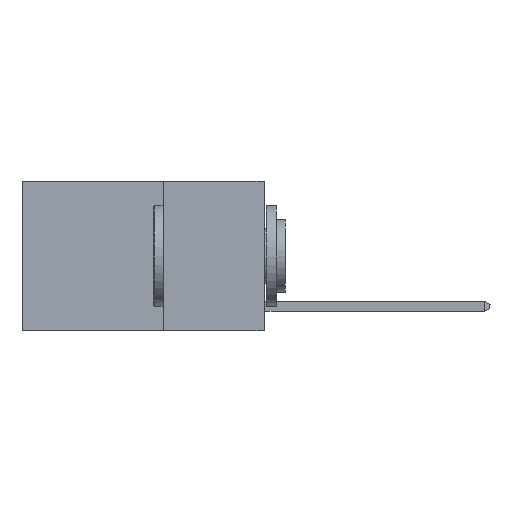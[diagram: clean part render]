
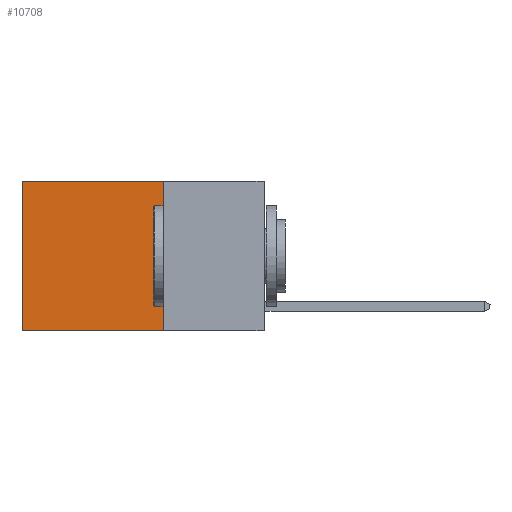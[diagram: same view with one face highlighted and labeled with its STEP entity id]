
A CAD part, left-side view. The second image highlights one B-rep face of the part: STEP entity #10708.
In plain terms, the highlighted planar face has unit normal (-1, 0, 0).
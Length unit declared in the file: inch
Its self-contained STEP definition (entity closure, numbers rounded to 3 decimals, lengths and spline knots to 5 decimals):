
#77 = LINE ( 'NONE', #4449, #6578 ) ;
#683 = DIRECTION ( 'NONE',  ( 0., 1., 0. ) ) ;
#2495 = PLANE ( 'NONE',  #8818 ) ;
#3598 = EDGE_CURVE ( 'NONE', #3905, #5558, #11132, .T. ) ;
#3905 = VERTEX_POINT ( 'NONE', #11980 ) ;
#4044 = CARTESIAN_POINT ( 'NONE',  ( 0.2625, 0.25, 0. ) ) ;
#4143 = DIRECTION ( 'NONE',  ( 0., 0., -1. ) ) ;
#4311 = EDGE_LOOP ( 'NONE', ( #5933, #10699, #9620, #6932 ) ) ;
#4449 = CARTESIAN_POINT ( 'NONE',  ( 0.2625, 0.6, 0. ) ) ;
#5146 = CARTESIAN_POINT ( 'NONE',  ( 0.2625, 0.25, -0.37 ) ) ;
#5380 = DIRECTION ( 'NONE',  ( 1., 0., 0. ) ) ;
#5442 = CARTESIAN_POINT ( 'NONE',  ( 0.2625, 0.6, 0. ) ) ;
#5558 = VERTEX_POINT ( 'NONE', #6359 ) ;
#5732 = DIRECTION ( 'NONE',  ( 0., 0., -1. ) ) ;
#5933 = ORIENTED_EDGE ( 'NONE', *, *, #17883, .T. ) ;
#6359 = CARTESIAN_POINT ( 'NONE',  ( 0.2625, 0.25, -0.37 ) ) ;
#6578 = VECTOR ( 'NONE', #5732, 39.37008 ) ;
#6932 = ORIENTED_EDGE ( 'NONE', *, *, #12185, .T. ) ;
#8719 = VECTOR ( 'NONE', #4143, 39.37008 ) ;
#8818 = AXIS2_PLACEMENT_3D ( 'NONE', #12377, #5380, #10980 ) ;
#9394 = VECTOR ( 'NONE', #683, 39.37008 ) ;
#9455 = VERTEX_POINT ( 'NONE', #5442 ) ;
#9460 = VECTOR ( 'NONE', #12829, 39.37008 ) ;
#9620 = ORIENTED_EDGE ( 'NONE', *, *, #3598, .F. ) ;
#9691 = EDGE_CURVE ( 'NONE', #5558, #10214, #13719, .T. ) ;
#9763 = CARTESIAN_POINT ( 'NONE',  ( 0.2625, 0.25, 0. ) ) ;
#10214 = VERTEX_POINT ( 'NONE', #15180 ) ;
#10699 = ORIENTED_EDGE ( 'NONE', *, *, #9691, .F. ) ;
#10708 = ADVANCED_FACE ( 'NONE', ( #12563 ), #2495, .F. ) ;
#10980 = DIRECTION ( 'NONE',  ( 0., 0., -1. ) ) ;
#11132 = LINE ( 'NONE', #4044, #8719 ) ;
#11980 = CARTESIAN_POINT ( 'NONE',  ( 0.2625, 0.25, 0. ) ) ;
#12185 = EDGE_CURVE ( 'NONE', #3905, #9455, #13935, .T. ) ;
#12377 = CARTESIAN_POINT ( 'NONE',  ( 0.2625, 0.25, 0. ) ) ;
#12563 = FACE_OUTER_BOUND ( 'NONE', #4311, .T. ) ;
#12829 = DIRECTION ( 'NONE',  ( 0., 1., 0. ) ) ;
#13719 = LINE ( 'NONE', #5146, #9394 ) ;
#13935 = LINE ( 'NONE', #9763, #9460 ) ;
#15180 = CARTESIAN_POINT ( 'NONE',  ( 0.2625, 0.6, -0.37 ) ) ;
#17883 = EDGE_CURVE ( 'NONE', #9455, #10214, #77, .T. ) ;
